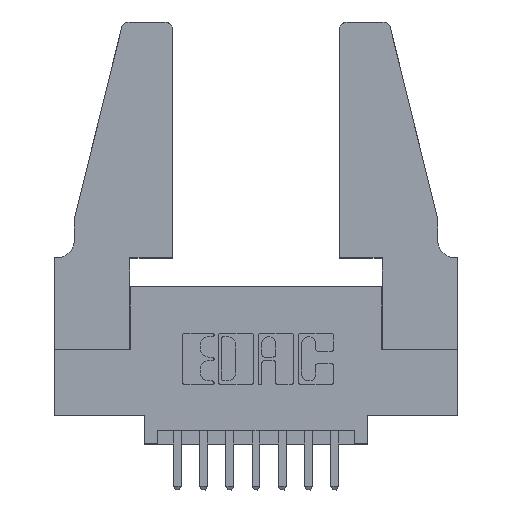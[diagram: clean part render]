
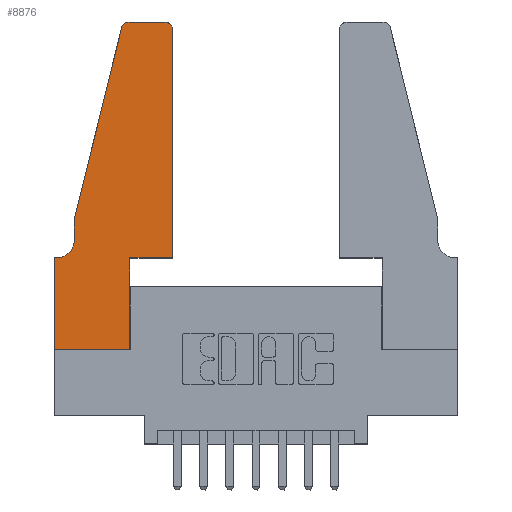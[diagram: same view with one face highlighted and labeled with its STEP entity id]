
A CAD part, top view. The second image highlights one B-rep face of the part: STEP entity #8876.
In plain terms, the highlighted planar face has unit normal (0, 0, 1).
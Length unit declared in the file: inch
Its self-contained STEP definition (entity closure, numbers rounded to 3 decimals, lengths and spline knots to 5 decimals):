
#87 = CIRCLE ( 'NONE', #8106, 0.03 ) ;
#186 = CARTESIAN_POINT ( 'NONE',  ( 0.4205, 1.22, 0.37 ) ) ;
#275 = DIRECTION ( 'NONE',  ( 1., 0., 0. ) ) ;
#291 = DIRECTION ( 'NONE',  ( -0.239, -0.971, 0. ) ) ;
#690 = ORIENTED_EDGE ( 'NONE', *, *, #5930, .T. ) ;
#791 = ORIENTED_EDGE ( 'NONE', *, *, #6026, .T. ) ;
#810 = VECTOR ( 'NONE', #10302, 39.37008 ) ;
#824 = EDGE_CURVE ( 'NONE', #9309, #10662, #9913, .T. ) ;
#1187 = DIRECTION ( 'NONE',  ( 1., 0., 0. ) ) ;
#1332 = LINE ( 'NONE', #9876, #6533 ) ;
#1477 = CARTESIAN_POINT ( 'NONE',  ( 0.0055, 0.42, 0.37 ) ) ;
#1509 = ORIENTED_EDGE ( 'NONE', *, *, #2190, .T. ) ;
#1914 = ORIENTED_EDGE ( 'NONE', *, *, #824, .T. ) ;
#2041 = LINE ( 'NONE', #9380, #12076 ) ;
#2088 = DIRECTION ( 'NONE',  ( 0., 1., 0. ) ) ;
#2125 = AXIS2_PLACEMENT_3D ( 'NONE', #8605, #9587, #3788 ) ;
#2190 = EDGE_CURVE ( 'NONE', #12383, #10784, #87, .T. ) ;
#2453 = VECTOR ( 'NONE', #275, 39.37008 ) ;
#2485 = VECTOR ( 'NONE', #6603, 39.37008 ) ;
#2491 = DIRECTION ( 'NONE',  ( -1., 0., 0. ) ) ;
#2501 = EDGE_CURVE ( 'NONE', #8388, #10141, #1332, .T. ) ;
#2644 = ORIENTED_EDGE ( 'NONE', *, *, #10362, .T. ) ;
#2706 = CARTESIAN_POINT ( 'NONE',  ( 0.0755, 0.5, 0.37 ) ) ;
#2796 = EDGE_CURVE ( 'NONE', #10170, #5254, #8635, .T. ) ;
#3274 = LINE ( 'NONE', #2706, #8123 ) ;
#3788 = DIRECTION ( 'NONE',  ( 1., 0., 0. ) ) ;
#4034 = CARTESIAN_POINT ( 'NONE',  ( 0.4505, 0.35, 0.37 ) ) ;
#4149 = ORIENTED_EDGE ( 'NONE', *, *, #2796, .T. ) ;
#4381 = AXIS2_PLACEMENT_3D ( 'NONE', #1477, #8297, #2491 ) ;
#4471 = LINE ( 'NONE', #11974, #11880 ) ;
#4561 = DIRECTION ( 'NONE',  ( -1., 0., 0. ) ) ;
#4588 = AXIS2_PLACEMENT_3D ( 'NONE', #186, #7045, #1187 ) ;
#4600 = DIRECTION ( 'NONE',  ( 0., 0., 1. ) ) ;
#4731 = ORIENTED_EDGE ( 'NONE', *, *, #5065, .T. ) ;
#4877 = CARTESIAN_POINT ( 'NONE',  ( 0.4505, 1.22, 0.37 ) ) ;
#5037 = LINE ( 'NONE', #7124, #2453 ) ;
#5065 = EDGE_CURVE ( 'NONE', #10141, #8544, #8738, .T. ) ;
#5109 = VECTOR ( 'NONE', #9269, 39.37008 ) ;
#5253 = CARTESIAN_POINT ( 'NONE',  ( 0.284, 1.25, 0.37 ) ) ;
#5254 = VERTEX_POINT ( 'NONE', #9241 ) ;
#5266 = VERTEX_POINT ( 'NONE', #8316 ) ;
#5299 = EDGE_CURVE ( 'NONE', #10662, #6315, #8594, .T. ) ;
#5314 = ORIENTED_EDGE ( 'NONE', *, *, #5875, .T. ) ;
#5487 = CARTESIAN_POINT ( 'NONE',  ( 0., 0., 0.37 ) ) ;
#5850 = ORIENTED_EDGE ( 'NONE', *, *, #2501, .T. ) ;
#5875 = EDGE_CURVE ( 'NONE', #8544, #12383, #7364, .T. ) ;
#5930 = EDGE_CURVE ( 'NONE', #6315, #6334, #9023, .T. ) ;
#6026 = EDGE_CURVE ( 'NONE', #5266, #10170, #3274, .T. ) ;
#6315 = VERTEX_POINT ( 'NONE', #7101 ) ;
#6334 = VERTEX_POINT ( 'NONE', #8076 ) ;
#6350 = CARTESIAN_POINT ( 'NONE',  ( 0., 0.35, 0.37 ) ) ;
#6470 = DIRECTION ( 'NONE',  ( 0., 1., 0. ) ) ;
#6533 = VECTOR ( 'NONE', #2088, 39.37008 ) ;
#6603 = DIRECTION ( 'NONE',  ( 0., -1., 0. ) ) ;
#6747 = CARTESIAN_POINT ( 'NONE',  ( 0.25487, 1.22718, 0.37 ) ) ;
#7045 = DIRECTION ( 'NONE',  ( 0., 0., 1. ) ) ;
#7101 = CARTESIAN_POINT ( 'NONE',  ( 0.2865, 0., 0.37 ) ) ;
#7124 = CARTESIAN_POINT ( 'NONE',  ( 0.4505, 0.35, 0.37 ) ) ;
#7364 = LINE ( 'NONE', #12155, #5109 ) ;
#7411 = EDGE_LOOP ( 'NONE', ( #5314, #1509, #2644, #791, #4149, #10580, #1914, #9494, #690, #9098, #5850, #4731 ) ) ;
#7558 = CARTESIAN_POINT ( 'NONE',  ( 0., 0., 0.37 ) ) ;
#7633 = PLANE ( 'NONE',  #2125 ) ;
#7818 = CARTESIAN_POINT ( 'NONE',  ( 0.0755, 0.42, 0.37 ) ) ;
#8076 = CARTESIAN_POINT ( 'NONE',  ( 0.2865, 0.35, 0.37 ) ) ;
#8106 = AXIS2_PLACEMENT_3D ( 'NONE', #10391, #4600, #11368 ) ;
#8123 = VECTOR ( 'NONE', #9481, 39.37008 ) ;
#8297 = DIRECTION ( 'NONE',  ( 0., 0., -1. ) ) ;
#8316 = CARTESIAN_POINT ( 'NONE',  ( 0.0755, 0.5, 0.37 ) ) ;
#8388 = VERTEX_POINT ( 'NONE', #4034 ) ;
#8544 = VERTEX_POINT ( 'NONE', #9074 ) ;
#8594 = LINE ( 'NONE', #5487, #810 ) ;
#8605 = CARTESIAN_POINT ( 'NONE',  ( 0., 0.35, 0.37 ) ) ;
#8635 = CIRCLE ( 'NONE', #4381, 0.07 ) ;
#8738 = CIRCLE ( 'NONE', #4588, 0.03 ) ;
#8746 = EDGE_CURVE ( 'NONE', #5254, #9309, #2041, .T. ) ;
#8876 = ADVANCED_FACE ( 'NONE', ( #10551 ), #7633, .T. ) ;
#9023 = LINE ( 'NONE', #11274, #12224 ) ;
#9074 = CARTESIAN_POINT ( 'NONE',  ( 0.4205, 1.25, 0.37 ) ) ;
#9098 = ORIENTED_EDGE ( 'NONE', *, *, #11645, .T. ) ;
#9241 = CARTESIAN_POINT ( 'NONE',  ( 0.0055, 0.35, 0.37 ) ) ;
#9269 = DIRECTION ( 'NONE',  ( -1., 0., 0. ) ) ;
#9309 = VERTEX_POINT ( 'NONE', #6350 ) ;
#9380 = CARTESIAN_POINT ( 'NONE',  ( 0.0755, 0.35, 0.37 ) ) ;
#9481 = DIRECTION ( 'NONE',  ( 0., -1., 0. ) ) ;
#9494 = ORIENTED_EDGE ( 'NONE', *, *, #5299, .T. ) ;
#9587 = DIRECTION ( 'NONE',  ( 0., 0., 1. ) ) ;
#9876 = CARTESIAN_POINT ( 'NONE',  ( 0.4505, 0.35, 0.37 ) ) ;
#9913 = LINE ( 'NONE', #9947, #2485 ) ;
#9947 = CARTESIAN_POINT ( 'NONE',  ( 0., 0., 0.37 ) ) ;
#10141 = VERTEX_POINT ( 'NONE', #4877 ) ;
#10170 = VERTEX_POINT ( 'NONE', #7818 ) ;
#10302 = DIRECTION ( 'NONE',  ( 1., 0., 0. ) ) ;
#10362 = EDGE_CURVE ( 'NONE', #10784, #5266, #4471, .T. ) ;
#10391 = CARTESIAN_POINT ( 'NONE',  ( 0.284, 1.22, 0.37 ) ) ;
#10551 = FACE_OUTER_BOUND ( 'NONE', #7411, .T. ) ;
#10580 = ORIENTED_EDGE ( 'NONE', *, *, #8746, .T. ) ;
#10662 = VERTEX_POINT ( 'NONE', #7558 ) ;
#10784 = VERTEX_POINT ( 'NONE', #6747 ) ;
#11274 = CARTESIAN_POINT ( 'NONE',  ( 0.2865, 0.35, 0.37 ) ) ;
#11368 = DIRECTION ( 'NONE',  ( 1., 0., 0. ) ) ;
#11645 = EDGE_CURVE ( 'NONE', #6334, #8388, #5037, .T. ) ;
#11880 = VECTOR ( 'NONE', #291, 39.37008 ) ;
#11974 = CARTESIAN_POINT ( 'NONE',  ( 0.0755, 0.5, 0.37 ) ) ;
#12076 = VECTOR ( 'NONE', #4561, 39.37008 ) ;
#12155 = CARTESIAN_POINT ( 'NONE',  ( 0.2605, 1.25, 0.37 ) ) ;
#12224 = VECTOR ( 'NONE', #6470, 39.37008 ) ;
#12383 = VERTEX_POINT ( 'NONE', #5253 ) ;
